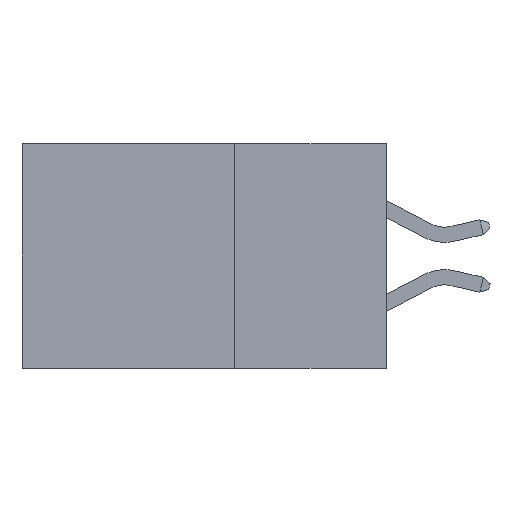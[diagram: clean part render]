
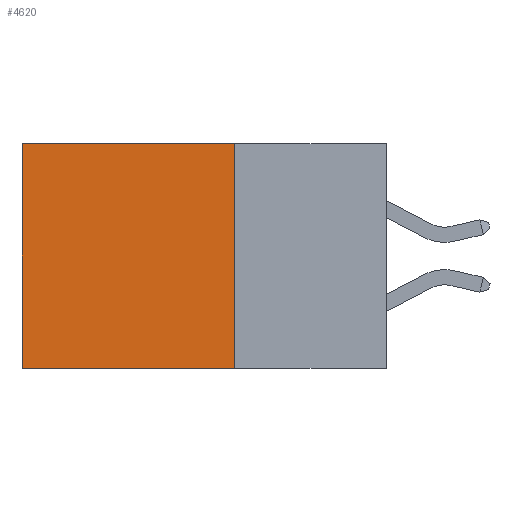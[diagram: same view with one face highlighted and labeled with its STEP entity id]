
A CAD part, left-side view. The second image highlights one B-rep face of the part: STEP entity #4620.
In plain terms, the highlighted planar face has unit normal (-1, 0, 0).
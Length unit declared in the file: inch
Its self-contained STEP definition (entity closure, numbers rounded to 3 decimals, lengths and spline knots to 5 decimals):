
#1068 = CARTESIAN_POINT ( 'NONE',  ( 0.298, 0.6, 0. ) ) ;
#1736 = CARTESIAN_POINT ( 'NONE',  ( 0.298, 0.25, 0. ) ) ;
#1785 = CARTESIAN_POINT ( 'NONE',  ( 0.298, 0.25, 0. ) ) ;
#2082 = VECTOR ( 'NONE', #4023, 39.37008 ) ;
#2319 = VERTEX_POINT ( 'NONE', #10637 ) ;
#2901 = VERTEX_POINT ( 'NONE', #15818 ) ;
#4023 = DIRECTION ( 'NONE',  ( 0., 0., -1. ) ) ;
#4620 = ADVANCED_FACE ( 'NONE', ( #14663 ), #7877, .F. ) ;
#4786 = EDGE_CURVE ( 'NONE', #2319, #2901, #10603, .T. ) ;
#4927 = EDGE_LOOP ( 'NONE', ( #6915, #16150, #10772, #17404 ) ) ;
#5709 = LINE ( 'NONE', #13557, #16179 ) ;
#5963 = CARTESIAN_POINT ( 'NONE',  ( 0.298, 0.25, 0. ) ) ;
#6915 = ORIENTED_EDGE ( 'NONE', *, *, #4786, .T. ) ;
#6993 = VECTOR ( 'NONE', #14170, 39.37008 ) ;
#7877 = PLANE ( 'NONE',  #18174 ) ;
#8039 = VERTEX_POINT ( 'NONE', #17119 ) ;
#8252 = VECTOR ( 'NONE', #17514, 39.37008 ) ;
#10276 = EDGE_CURVE ( 'NONE', #14221, #2319, #13617, .T. ) ;
#10603 = LINE ( 'NONE', #1068, #6993 ) ;
#10637 = CARTESIAN_POINT ( 'NONE',  ( 0.298, 0.6, 0. ) ) ;
#10772 = ORIENTED_EDGE ( 'NONE', *, *, #10885, .F. ) ;
#10806 = LINE ( 'NONE', #12168, #2082 ) ;
#10885 = EDGE_CURVE ( 'NONE', #14221, #8039, #10806, .T. ) ;
#12168 = CARTESIAN_POINT ( 'NONE',  ( 0.298, 0.25, 0. ) ) ;
#13557 = CARTESIAN_POINT ( 'NONE',  ( 0.298, 0.25, -0.37 ) ) ;
#13617 = LINE ( 'NONE', #5963, #8252 ) ;
#14170 = DIRECTION ( 'NONE',  ( 0., 0., -1. ) ) ;
#14221 = VERTEX_POINT ( 'NONE', #1736 ) ;
#14246 = DIRECTION ( 'NONE',  ( 1., 0., 0. ) ) ;
#14663 = FACE_OUTER_BOUND ( 'NONE', #4927, .T. ) ;
#14916 = DIRECTION ( 'NONE',  ( 0., 1., 0. ) ) ;
#15818 = CARTESIAN_POINT ( 'NONE',  ( 0.298, 0.6, -0.37 ) ) ;
#16150 = ORIENTED_EDGE ( 'NONE', *, *, #18833, .F. ) ;
#16179 = VECTOR ( 'NONE', #14916, 39.37008 ) ;
#16373 = DIRECTION ( 'NONE',  ( 0., 0., -1. ) ) ;
#17119 = CARTESIAN_POINT ( 'NONE',  ( 0.298, 0.25, -0.37 ) ) ;
#17404 = ORIENTED_EDGE ( 'NONE', *, *, #10276, .T. ) ;
#17514 = DIRECTION ( 'NONE',  ( 0., 1., 0. ) ) ;
#18174 = AXIS2_PLACEMENT_3D ( 'NONE', #1785, #14246, #16373 ) ;
#18833 = EDGE_CURVE ( 'NONE', #8039, #2901, #5709, .T. ) ;
